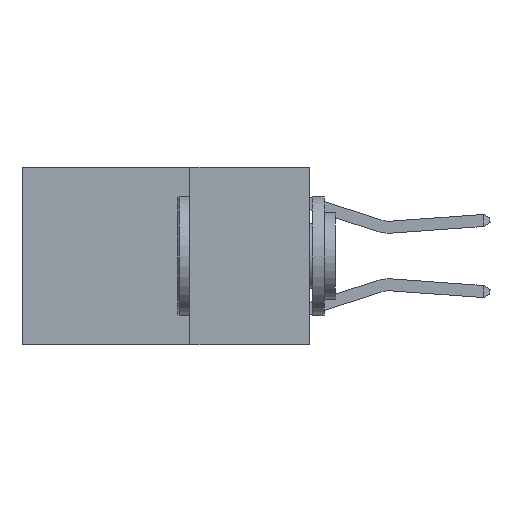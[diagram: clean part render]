
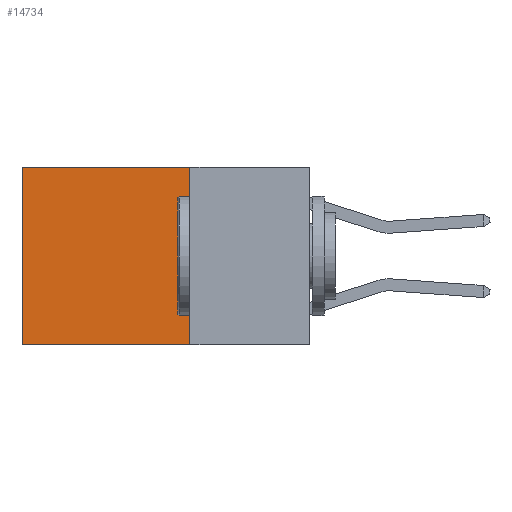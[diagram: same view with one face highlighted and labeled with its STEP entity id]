
A CAD part, left-side view. The second image highlights one B-rep face of the part: STEP entity #14734.
In plain terms, the highlighted planar face has unit normal (-1, 0, 0).
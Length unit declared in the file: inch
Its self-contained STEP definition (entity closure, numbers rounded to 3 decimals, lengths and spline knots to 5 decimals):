
#611 = DIRECTION ( 'NONE',  ( 1., 0., 0. ) ) ;
#1683 = LINE ( 'NONE', #2798, #3816 ) ;
#1965 = VERTEX_POINT ( 'NONE', #6781 ) ;
#2798 = CARTESIAN_POINT ( 'NONE',  ( 0.2625, 0.6, 0. ) ) ;
#2821 = AXIS2_PLACEMENT_3D ( 'NONE', #18851, #611, #5037 ) ;
#2927 = EDGE_CURVE ( 'NONE', #4378, #17980, #5313, .T. ) ;
#3147 = CARTESIAN_POINT ( 'NONE',  ( 0.2625, 0.25, 0. ) ) ;
#3807 = DIRECTION ( 'NONE',  ( 0., 1., 0. ) ) ;
#3816 = VECTOR ( 'NONE', #7428, 39.37008 ) ;
#4378 = VERTEX_POINT ( 'NONE', #8654 ) ;
#4941 = DIRECTION ( 'NONE',  ( 0., 0., -1. ) ) ;
#5037 = DIRECTION ( 'NONE',  ( 0., 0., -1. ) ) ;
#5219 = DIRECTION ( 'NONE',  ( 0., 1., 0. ) ) ;
#5242 = VECTOR ( 'NONE', #3807, 39.37008 ) ;
#5313 = LINE ( 'NONE', #17534, #5242 ) ;
#5714 = EDGE_CURVE ( 'NONE', #1965, #19016, #19045, .T. ) ;
#6045 = ORIENTED_EDGE ( 'NONE', *, *, #12509, .T. ) ;
#6781 = CARTESIAN_POINT ( 'NONE',  ( 0.2625, 0.25, 0. ) ) ;
#7428 = DIRECTION ( 'NONE',  ( 0., 0., -1. ) ) ;
#7462 = ORIENTED_EDGE ( 'NONE', *, *, #5714, .T. ) ;
#7846 = CARTESIAN_POINT ( 'NONE',  ( 0.2625, 0.6, 0. ) ) ;
#7863 = VECTOR ( 'NONE', #5219, 39.37008 ) ;
#8267 = PLANE ( 'NONE',  #2821 ) ;
#8654 = CARTESIAN_POINT ( 'NONE',  ( 0.2625, 0.25, -0.37 ) ) ;
#9349 = VECTOR ( 'NONE', #4941, 39.37008 ) ;
#9582 = LINE ( 'NONE', #3147, #9349 ) ;
#11361 = FACE_OUTER_BOUND ( 'NONE', #16797, .T. ) ;
#12224 = CARTESIAN_POINT ( 'NONE',  ( 0.2625, 0.6, -0.37 ) ) ;
#12509 = EDGE_CURVE ( 'NONE', #19016, #17980, #1683, .T. ) ;
#13187 = CARTESIAN_POINT ( 'NONE',  ( 0.2625, 0.25, 0. ) ) ;
#14734 = ADVANCED_FACE ( 'NONE', ( #11361 ), #8267, .F. ) ;
#16797 = EDGE_LOOP ( 'NONE', ( #6045, #16813, #18278, #7462 ) ) ;
#16813 = ORIENTED_EDGE ( 'NONE', *, *, #2927, .F. ) ;
#17534 = CARTESIAN_POINT ( 'NONE',  ( 0.2625, 0.25, -0.37 ) ) ;
#17980 = VERTEX_POINT ( 'NONE', #12224 ) ;
#18278 = ORIENTED_EDGE ( 'NONE', *, *, #18539, .F. ) ;
#18539 = EDGE_CURVE ( 'NONE', #1965, #4378, #9582, .T. ) ;
#18851 = CARTESIAN_POINT ( 'NONE',  ( 0.2625, 0.25, 0. ) ) ;
#19016 = VERTEX_POINT ( 'NONE', #7846 ) ;
#19045 = LINE ( 'NONE', #13187, #7863 ) ;
